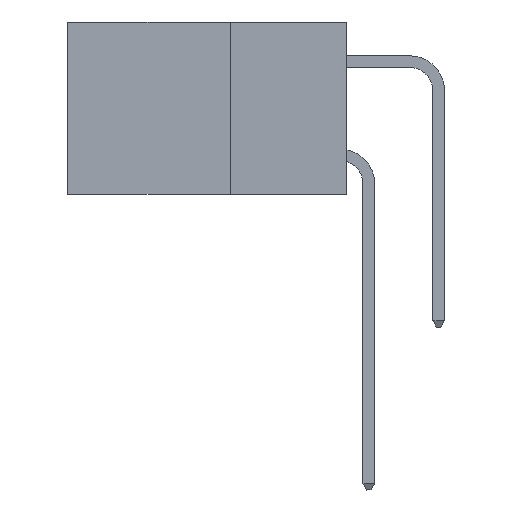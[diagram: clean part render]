
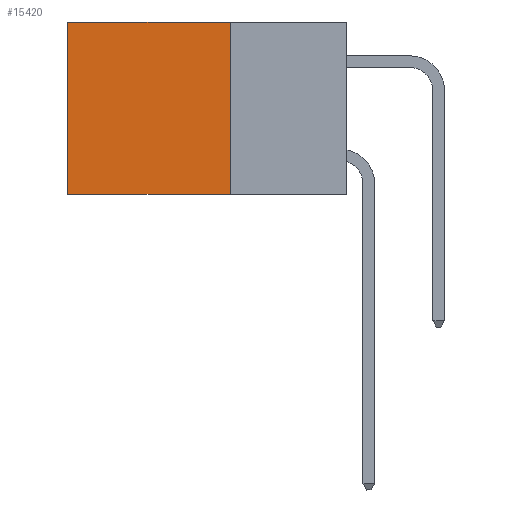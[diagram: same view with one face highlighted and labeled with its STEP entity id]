
A CAD part, left-side view. The second image highlights one B-rep face of the part: STEP entity #15420.
In plain terms, the highlighted planar face has unit normal (-1, 0, 0).
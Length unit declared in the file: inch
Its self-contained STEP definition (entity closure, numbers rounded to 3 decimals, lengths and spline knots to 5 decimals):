
#233 = AXIS2_PLACEMENT_3D ( 'NONE', #39582, #33538, #33415 ) ;
#2172 = CARTESIAN_POINT ( 'NONE',  ( 0.2875, 0.6, 0. ) ) ;
#5404 = CARTESIAN_POINT ( 'NONE',  ( 0.2875, 0.25, 0. ) ) ;
#10238 = LINE ( 'NONE', #5404, #21844 ) ;
#11092 = EDGE_LOOP ( 'NONE', ( #17379, #25341, #13416, #18784 ) ) ;
#11563 = LINE ( 'NONE', #2172, #27981 ) ;
#11847 = PLANE ( 'NONE',  #233 ) ;
#12690 = DIRECTION ( 'NONE',  ( 0., 1., 0. ) ) ;
#13416 = ORIENTED_EDGE ( 'NONE', *, *, #38411, .F. ) ;
#13755 = CARTESIAN_POINT ( 'NONE',  ( 0.2875, 0.6, -0.37 ) ) ;
#14547 = DIRECTION ( 'NONE',  ( 0., 1., 0. ) ) ;
#15420 = ADVANCED_FACE ( 'NONE', ( #29572 ), #11847, .F. ) ;
#16091 = VERTEX_POINT ( 'NONE', #26776 ) ;
#16545 = LINE ( 'NONE', #24955, #30515 ) ;
#16725 = VECTOR ( 'NONE', #37810, 39.37008 ) ;
#17379 = ORIENTED_EDGE ( 'NONE', *, *, #36637, .T. ) ;
#18784 = ORIENTED_EDGE ( 'NONE', *, *, #28966, .T. ) ;
#21192 = CARTESIAN_POINT ( 'NONE',  ( 0.2875, 0.25, 0. ) ) ;
#21844 = VECTOR ( 'NONE', #14547, 39.37008 ) ;
#23534 = DIRECTION ( 'NONE',  ( 0., 0., -1. ) ) ;
#24226 = EDGE_CURVE ( 'NONE', #16091, #39645, #16545, .T. ) ;
#24955 = CARTESIAN_POINT ( 'NONE',  ( 0.2875, 0.25, -0.37 ) ) ;
#25341 = ORIENTED_EDGE ( 'NONE', *, *, #24226, .F. ) ;
#25835 = CARTESIAN_POINT ( 'NONE',  ( 0.2875, 0.25, 0. ) ) ;
#26776 = CARTESIAN_POINT ( 'NONE',  ( 0.2875, 0.25, -0.37 ) ) ;
#27981 = VECTOR ( 'NONE', #23534, 39.37008 ) ;
#28966 = EDGE_CURVE ( 'NONE', #31840, #32615, #10238, .T. ) ;
#29572 = FACE_OUTER_BOUND ( 'NONE', #11092, .T. ) ;
#30515 = VECTOR ( 'NONE', #12690, 39.37008 ) ;
#31840 = VERTEX_POINT ( 'NONE', #21192 ) ;
#32615 = VERTEX_POINT ( 'NONE', #34218 ) ;
#33415 = DIRECTION ( 'NONE',  ( 0., 0., -1. ) ) ;
#33538 = DIRECTION ( 'NONE',  ( 1., 0., 0. ) ) ;
#34218 = CARTESIAN_POINT ( 'NONE',  ( 0.2875, 0.6, 0. ) ) ;
#36637 = EDGE_CURVE ( 'NONE', #32615, #39645, #11563, .T. ) ;
#37810 = DIRECTION ( 'NONE',  ( 0., 0., -1. ) ) ;
#37886 = LINE ( 'NONE', #25835, #16725 ) ;
#38411 = EDGE_CURVE ( 'NONE', #31840, #16091, #37886, .T. ) ;
#39582 = CARTESIAN_POINT ( 'NONE',  ( 0.2875, 0.25, 0. ) ) ;
#39645 = VERTEX_POINT ( 'NONE', #13755 ) ;
